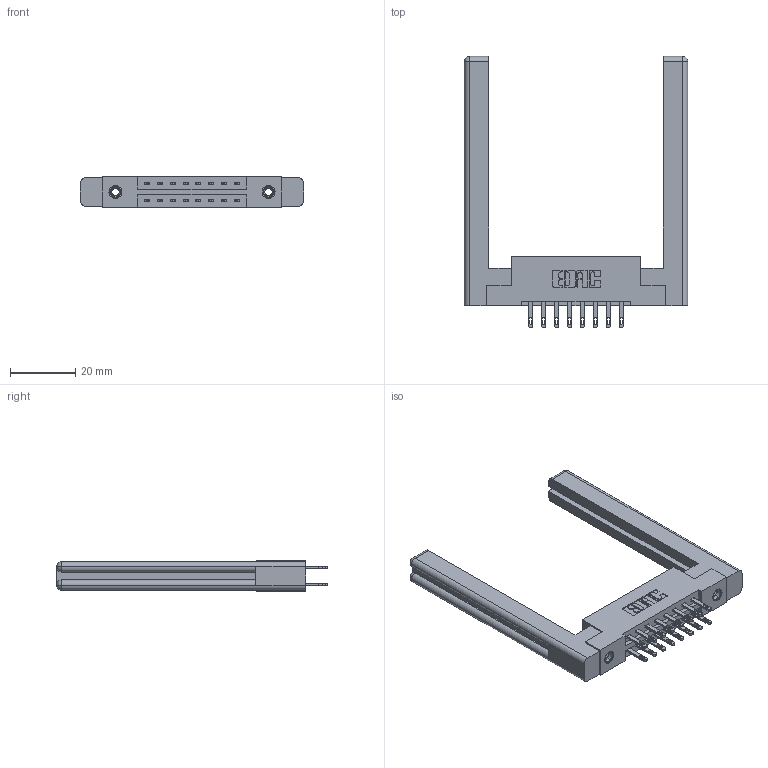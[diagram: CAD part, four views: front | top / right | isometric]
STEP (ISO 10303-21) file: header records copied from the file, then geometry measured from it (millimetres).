
FILE_DESCRIPTION (( 'STEP AP203' ), '1' );
FILE_NAME ('337-016-500-258.STEP', '2019-10-08T12:10:59', ( '' ), ( '' ), 'SwSTEP 2.0', 'SolidWorks 2016', '' );
FILE_SCHEMA (( 'CONFIG_CONTROL_DESIGN' ));
Length unit declared in the file: inch
Products named in the file (5): 307-220-058; 337-016-500-258; 345-250-001_345-250-001-102; 337 Part_Flush Mounting Lugs - 0.156 Dia-TI; 345-292-001_345-293-100
Assembly tree (21 placements, depth 2):
  337-016-500-258
    337 Part_Flush Mounting Lugs - 0.156 Dia-TI
    345-292-001_345-293-100  x16
    345-250-001_345-250-001-102  x2
    307-220-058  x2
Bounding box: 68.33 x 82.94 x 9.4 mm (x, y, z)
Volume: 13939.4 mm3; surface area: 12578.1 mm2
Topology: 21 solids, 21 shells, 1056 faces, 3113 edges, 2062 vertices
Faces by surface type: plane 666, cylinder 366, cone 12, torus 12
Entity records: 13164 total; most frequent: CARTESIAN_POINT 2253, ORIENTED_EDGE 2128, DIRECTION 1996, EDGE_CURVE 1064, VECTOR 884, LINE 884, VERTEX_POINT 702, AXIS2_PLACEMENT_3D 556
